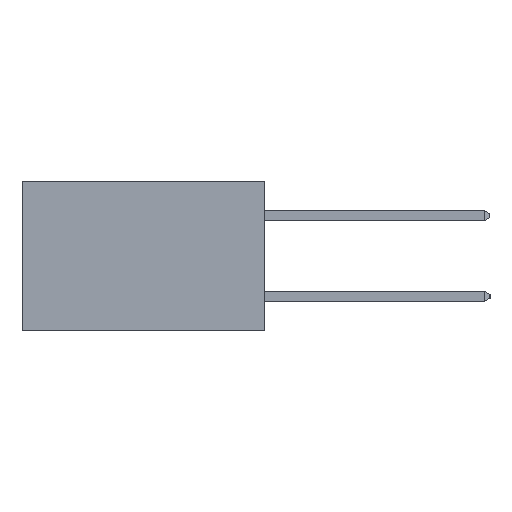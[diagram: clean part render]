
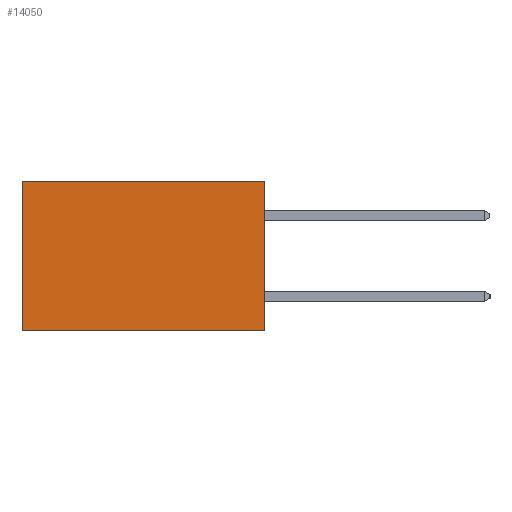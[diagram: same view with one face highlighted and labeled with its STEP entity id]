
A CAD part, left-side view. The second image highlights one B-rep face of the part: STEP entity #14050.
In plain terms, the highlighted planar face has unit normal (-1, 0, 0).
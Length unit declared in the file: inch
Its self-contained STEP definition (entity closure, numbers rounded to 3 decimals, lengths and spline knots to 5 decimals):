
#28 = EDGE_CURVE ( 'NONE', #17516, #15751, #15496, .T. ) ;
#653 = VECTOR ( 'NONE', #7137, 39.37008 ) ;
#1205 = ORIENTED_EDGE ( 'NONE', *, *, #28, .F. ) ;
#1213 = ORIENTED_EDGE ( 'NONE', *, *, #11639, .T. ) ;
#1482 = DIRECTION ( 'NONE',  ( 0., 0., -1. ) ) ;
#1855 = CARTESIAN_POINT ( 'NONE',  ( 0.2615, 0., -0.37 ) ) ;
#2328 = CARTESIAN_POINT ( 'NONE',  ( 0.2615, 0., -0.37 ) ) ;
#3630 = EDGE_CURVE ( 'NONE', #3717, #17516, #7662, .T. ) ;
#3717 = VERTEX_POINT ( 'NONE', #12821 ) ;
#5641 = DIRECTION ( 'NONE',  ( 0., 1., 0. ) ) ;
#5905 = CARTESIAN_POINT ( 'NONE',  ( 0.2615, 0.6, -0.37 ) ) ;
#6292 = VERTEX_POINT ( 'NONE', #10522 ) ;
#6379 = VECTOR ( 'NONE', #1482, 39.37008 ) ;
#7137 = DIRECTION ( 'NONE',  ( 0., 1., 0. ) ) ;
#7225 = VECTOR ( 'NONE', #11881, 39.37008 ) ;
#7662 = LINE ( 'NONE', #11631, #7225 ) ;
#7744 = DIRECTION ( 'NONE',  ( 0., 0., -1. ) ) ;
#9916 = FACE_OUTER_BOUND ( 'NONE', #17339, .T. ) ;
#10522 = CARTESIAN_POINT ( 'NONE',  ( 0.2615, 0.6, 0. ) ) ;
#11631 = CARTESIAN_POINT ( 'NONE',  ( 0.2615, 0., -0.37 ) ) ;
#11639 = EDGE_CURVE ( 'NONE', #3717, #6292, #12836, .T. ) ;
#11881 = DIRECTION ( 'NONE',  ( 0., 0., -1. ) ) ;
#11895 = CARTESIAN_POINT ( 'NONE',  ( 0.2615, 0., -0.37 ) ) ;
#12701 = CARTESIAN_POINT ( 'NONE',  ( 0.2615, 0.6, -0.37 ) ) ;
#12821 = CARTESIAN_POINT ( 'NONE',  ( 0.2615, 0., 0. ) ) ;
#12836 = LINE ( 'NONE', #13976, #13261 ) ;
#13261 = VECTOR ( 'NONE', #5641, 39.37008 ) ;
#13976 = CARTESIAN_POINT ( 'NONE',  ( 0.2615, 0., 0. ) ) ;
#14050 = ADVANCED_FACE ( 'NONE', ( #9916 ), #14645, .F. ) ;
#14261 = ORIENTED_EDGE ( 'NONE', *, *, #3630, .F. ) ;
#14645 = PLANE ( 'NONE',  #15431 ) ;
#15123 = EDGE_CURVE ( 'NONE', #6292, #15751, #17778, .T. ) ;
#15431 = AXIS2_PLACEMENT_3D ( 'NONE', #11895, #15949, #7744 ) ;
#15496 = LINE ( 'NONE', #2328, #653 ) ;
#15528 = ORIENTED_EDGE ( 'NONE', *, *, #15123, .T. ) ;
#15751 = VERTEX_POINT ( 'NONE', #5905 ) ;
#15949 = DIRECTION ( 'NONE',  ( 1., 0., 0. ) ) ;
#17339 = EDGE_LOOP ( 'NONE', ( #15528, #1205, #14261, #1213 ) ) ;
#17516 = VERTEX_POINT ( 'NONE', #1855 ) ;
#17778 = LINE ( 'NONE', #12701, #6379 ) ;
